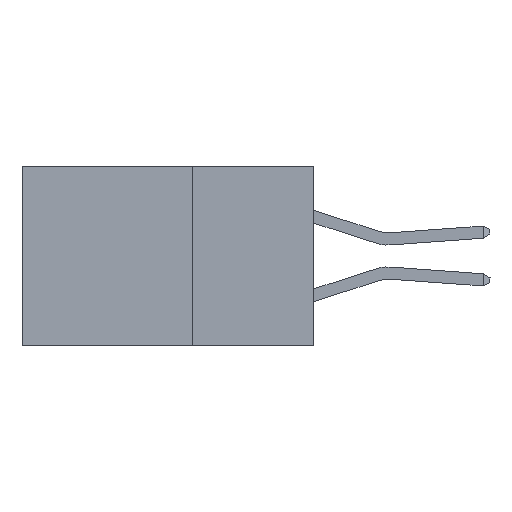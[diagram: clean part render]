
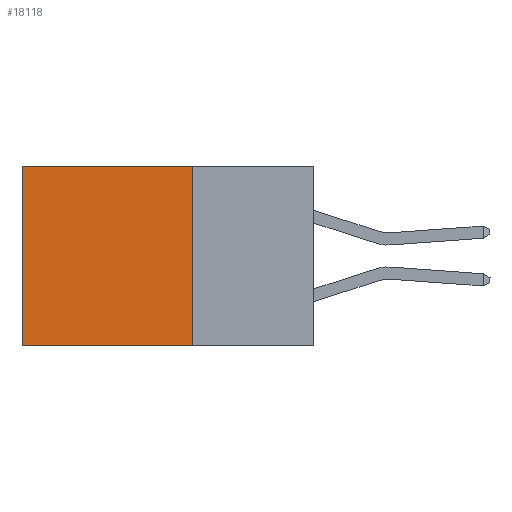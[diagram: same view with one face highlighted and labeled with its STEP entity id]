
A CAD part, left-side view. The second image highlights one B-rep face of the part: STEP entity #18118.
In plain terms, the highlighted planar face has unit normal (-1, 0, 0).
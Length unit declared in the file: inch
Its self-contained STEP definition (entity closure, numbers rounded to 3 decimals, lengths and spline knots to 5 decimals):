
#1747 = FACE_OUTER_BOUND ( 'NONE', #29008, .T. ) ;
#1898 = VECTOR ( 'NONE', #42526, 39.37008 ) ;
#2552 = LINE ( 'NONE', #36397, #15961 ) ;
#3094 = DIRECTION ( 'NONE',  ( 0., 0., -1. ) ) ;
#4150 = CARTESIAN_POINT ( 'NONE',  ( 0.2875, 0.6, 0. ) ) ;
#5601 = ORIENTED_EDGE ( 'NONE', *, *, #11211, .T. ) ;
#6479 = ORIENTED_EDGE ( 'NONE', *, *, #23878, .F. ) ;
#7026 = ORIENTED_EDGE ( 'NONE', *, *, #12579, .T. ) ;
#7836 = EDGE_CURVE ( 'NONE', #28503, #25688, #37655, .T. ) ;
#8376 = VECTOR ( 'NONE', #19246, 39.37008 ) ;
#11096 = DIRECTION ( 'NONE',  ( 0., 0., -1. ) ) ;
#11211 = EDGE_CURVE ( 'NONE', #28503, #22554, #17122, .T. ) ;
#12579 = EDGE_CURVE ( 'NONE', #22554, #33147, #2552, .T. ) ;
#15961 = VECTOR ( 'NONE', #3094, 39.37008 ) ;
#17122 = LINE ( 'NONE', #22992, #8376 ) ;
#17979 = DIRECTION ( 'NONE',  ( 0., 1., 0. ) ) ;
#18118 = ADVANCED_FACE ( 'NONE', ( #1747 ), #40481, .F. ) ;
#19246 = DIRECTION ( 'NONE',  ( 0., 1., 0. ) ) ;
#19823 = LINE ( 'NONE', #27536, #21893 ) ;
#20607 = CARTESIAN_POINT ( 'NONE',  ( 0.2875, 0.25, 0. ) ) ;
#20892 = DIRECTION ( 'NONE',  ( 1., 0., 0. ) ) ;
#21893 = VECTOR ( 'NONE', #17979, 39.37008 ) ;
#22554 = VERTEX_POINT ( 'NONE', #4150 ) ;
#22992 = CARTESIAN_POINT ( 'NONE',  ( 0.2875, 0.25, 0. ) ) ;
#23878 = EDGE_CURVE ( 'NONE', #25688, #33147, #19823, .T. ) ;
#24487 = AXIS2_PLACEMENT_3D ( 'NONE', #20607, #20892, #11096 ) ;
#25688 = VERTEX_POINT ( 'NONE', #34193 ) ;
#27536 = CARTESIAN_POINT ( 'NONE',  ( 0.2875, 0.25, -0.37 ) ) ;
#28161 = ORIENTED_EDGE ( 'NONE', *, *, #7836, .F. ) ;
#28503 = VERTEX_POINT ( 'NONE', #33795 ) ;
#29008 = EDGE_LOOP ( 'NONE', ( #7026, #6479, #28161, #5601 ) ) ;
#33147 = VERTEX_POINT ( 'NONE', #38743 ) ;
#33795 = CARTESIAN_POINT ( 'NONE',  ( 0.2875, 0.25, 0. ) ) ;
#34193 = CARTESIAN_POINT ( 'NONE',  ( 0.2875, 0.25, -0.37 ) ) ;
#35870 = CARTESIAN_POINT ( 'NONE',  ( 0.2875, 0.25, 0. ) ) ;
#36397 = CARTESIAN_POINT ( 'NONE',  ( 0.2875, 0.6, 0. ) ) ;
#37655 = LINE ( 'NONE', #35870, #1898 ) ;
#38743 = CARTESIAN_POINT ( 'NONE',  ( 0.2875, 0.6, -0.37 ) ) ;
#40481 = PLANE ( 'NONE',  #24487 ) ;
#42526 = DIRECTION ( 'NONE',  ( 0., 0., -1. ) ) ;
